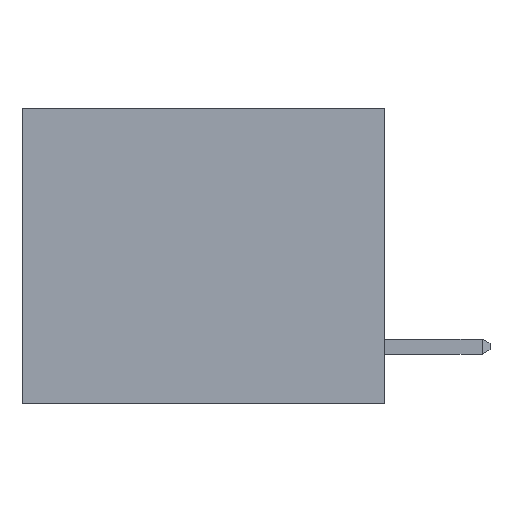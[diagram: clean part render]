
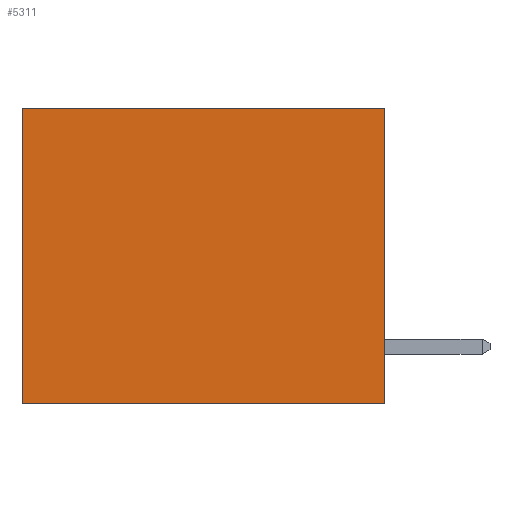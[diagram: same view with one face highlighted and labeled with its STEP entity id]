
A CAD part, left-side view. The second image highlights one B-rep face of the part: STEP entity #5311.
In plain terms, the highlighted planar face has unit normal (-1, 0, 0).
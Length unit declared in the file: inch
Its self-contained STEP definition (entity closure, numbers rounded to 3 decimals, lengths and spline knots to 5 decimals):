
#359 = CARTESIAN_POINT ( 'NONE',  ( 0.3165, 0., 0. ) ) ;
#654 = EDGE_LOOP ( 'NONE', ( #5754, #1630, #5949, #1707 ) ) ;
#834 = CARTESIAN_POINT ( 'NONE',  ( 0.3165, 0., -0.49 ) ) ;
#910 = DIRECTION ( 'NONE',  ( 1., 0., 0. ) ) ;
#1469 = CARTESIAN_POINT ( 'NONE',  ( 0.3165, 0.6, -0.49 ) ) ;
#1630 = ORIENTED_EDGE ( 'NONE', *, *, #10175, .F. ) ;
#1707 = ORIENTED_EDGE ( 'NONE', *, *, #4823, .T. ) ;
#2108 = LINE ( 'NONE', #9076, #7148 ) ;
#3221 = EDGE_CURVE ( 'NONE', #4408, #7187, #9366, .T. ) ;
#3277 = DIRECTION ( 'NONE',  ( 0., 0., -1. ) ) ;
#3599 = LINE ( 'NONE', #834, #4979 ) ;
#4076 = CARTESIAN_POINT ( 'NONE',  ( 0.3165, 0., -0.49 ) ) ;
#4408 = VERTEX_POINT ( 'NONE', #9164 ) ;
#4629 = VERTEX_POINT ( 'NONE', #6413 ) ;
#4705 = DIRECTION ( 'NONE',  ( 0., 0., -1. ) ) ;
#4823 = EDGE_CURVE ( 'NONE', #6366, #4408, #2108, .T. ) ;
#4845 = DIRECTION ( 'NONE',  ( 0., 0., -1. ) ) ;
#4979 = VECTOR ( 'NONE', #3277, 39.37008 ) ;
#5311 = ADVANCED_FACE ( 'NONE', ( #8937 ), #6542, .F. ) ;
#5754 = ORIENTED_EDGE ( 'NONE', *, *, #3221, .T. ) ;
#5949 = ORIENTED_EDGE ( 'NONE', *, *, #8539, .F. ) ;
#6316 = VECTOR ( 'NONE', #6697, 39.37008 ) ;
#6366 = VERTEX_POINT ( 'NONE', #359 ) ;
#6413 = CARTESIAN_POINT ( 'NONE',  ( 0.3165, 0., -0.49 ) ) ;
#6542 = PLANE ( 'NONE',  #9536 ) ;
#6680 = DIRECTION ( 'NONE',  ( 0., 1., 0. ) ) ;
#6697 = DIRECTION ( 'NONE',  ( 0., 1., 0. ) ) ;
#6817 = LINE ( 'NONE', #9965, #6316 ) ;
#7148 = VECTOR ( 'NONE', #6680, 39.37008 ) ;
#7187 = VERTEX_POINT ( 'NONE', #10283 ) ;
#8539 = EDGE_CURVE ( 'NONE', #6366, #4629, #3599, .T. ) ;
#8937 = FACE_OUTER_BOUND ( 'NONE', #654, .T. ) ;
#9076 = CARTESIAN_POINT ( 'NONE',  ( 0.3165, 0., 0. ) ) ;
#9164 = CARTESIAN_POINT ( 'NONE',  ( 0.3165, 0.6, 0. ) ) ;
#9366 = LINE ( 'NONE', #1469, #10118 ) ;
#9536 = AXIS2_PLACEMENT_3D ( 'NONE', #4076, #910, #4845 ) ;
#9965 = CARTESIAN_POINT ( 'NONE',  ( 0.3165, 0., -0.49 ) ) ;
#10118 = VECTOR ( 'NONE', #4705, 39.37008 ) ;
#10175 = EDGE_CURVE ( 'NONE', #4629, #7187, #6817, .T. ) ;
#10283 = CARTESIAN_POINT ( 'NONE',  ( 0.3165, 0.6, -0.49 ) ) ;
